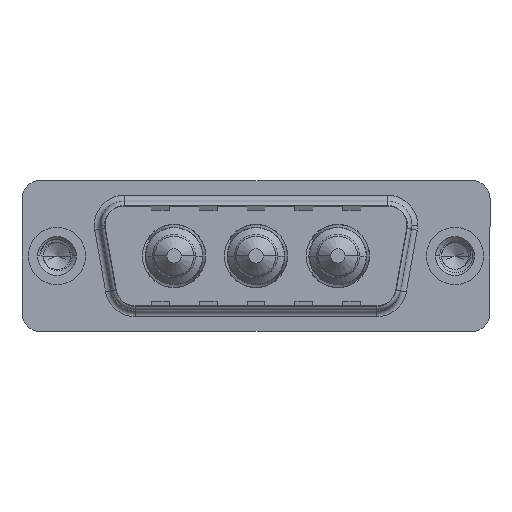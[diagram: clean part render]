
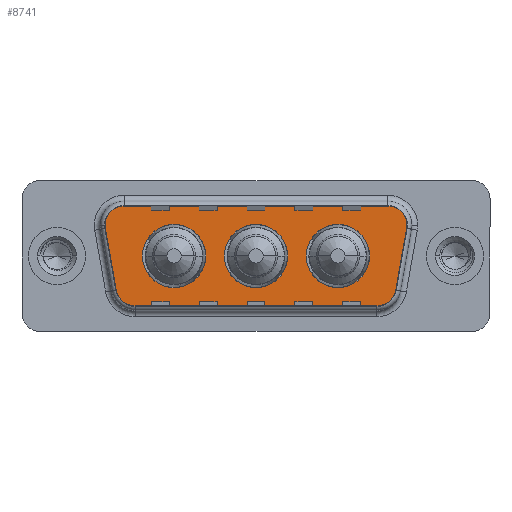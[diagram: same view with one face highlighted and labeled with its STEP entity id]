
A CAD part, top view. The second image highlights one B-rep face of the part: STEP entity #8741.
In plain terms, the highlighted planar face has unit normal (0, 0, 1).
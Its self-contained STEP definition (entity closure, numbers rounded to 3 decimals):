
#190 = CARTESIAN_POINT ( 'NONE',  ( 19.3, 0., 0. ) ) ;
#378 = DIRECTION ( 'NONE',  ( 1., 0., 0. ) ) ;
#458 = ORIENTED_EDGE ( 'NONE', *, *, #9914, .T. ) ;
#621 = VERTEX_POINT ( 'NONE', #1426 ) ;
#658 = LINE ( 'NONE', #4299, #10879 ) ;
#690 = DIRECTION ( 'NONE',  ( 0.174, -0.985, 0. ) ) ;
#710 = CARTESIAN_POINT ( 'NONE',  ( 16.65, 0., 0. ) ) ;
#801 = CARTESIAN_POINT ( 'NONE',  ( 5.411, 2.9, 0. ) ) ;
#1151 = CARTESIAN_POINT ( 'NONE',  ( 26.866, -2.9, 0. ) ) ;
#1298 = AXIS2_PLACEMENT_3D ( 'NONE', #11252, #2921, #12631 ) ;
#1360 = VECTOR ( 'NONE', #6233, 1000. ) ;
#1426 = CARTESIAN_POINT ( 'NONE',  ( 3.441, 2.553, 0. ) ) ;
#1449 = CARTESIAN_POINT ( 'NONE',  ( 27.889, 2.9, 0. ) ) ;
#1453 = VERTEX_POINT ( 'NONE', #14116 ) ;
#1493 = EDGE_CURVE ( 'NONE', #16702, #14204, #7532, .T. ) ;
#1863 = LINE ( 'NONE', #9044, #16305 ) ;
#2009 = CIRCLE ( 'NONE', #5411, 2.65 ) ;
#2084 = CARTESIAN_POINT ( 'NONE',  ( 16.65, 0., 0. ) ) ;
#2113 = ORIENTED_EDGE ( 'NONE', *, *, #17236, .T. ) ;
#2204 = DIRECTION ( 'NONE',  ( 1., 0., 0. ) ) ;
#2831 = DIRECTION ( 'NONE',  ( -1., 0., 0. ) ) ;
#2879 = VERTEX_POINT ( 'NONE', #17013 ) ;
#2913 = AXIS2_PLACEMENT_3D ( 'NONE', #4550, #14225, #5935 ) ;
#2921 = DIRECTION ( 'NONE',  ( 0., 0., 1. ) ) ;
#3236 = CARTESIAN_POINT ( 'NONE',  ( 4.464, -3.247, 0. ) ) ;
#3261 = ORIENTED_EDGE ( 'NONE', *, *, #8033, .T. ) ;
#3480 = AXIS2_PLACEMENT_3D ( 'NONE', #12303, #3997, #13688 ) ;
#3515 = CIRCLE ( 'NONE', #6598, 2. ) ;
#3562 = AXIS2_PLACEMENT_3D ( 'NONE', #13715, #13669, #4082 ) ;
#3754 = ORIENTED_EDGE ( 'NONE', *, *, #13810, .T. ) ;
#3919 = FACE_BOUND ( 'NONE', #4294, .T. ) ;
#3942 = DIRECTION ( 'NONE',  ( 1., 0., 0. ) ) ;
#3997 = DIRECTION ( 'NONE',  ( 0., 0., 1. ) ) ;
#4053 = CIRCLE ( 'NONE', #2913, 2.65 ) ;
#4074 = ORIENTED_EDGE ( 'NONE', *, *, #1493, .F. ) ;
#4082 = DIRECTION ( 'NONE',  ( -1., 0., 0. ) ) ;
#4184 = CARTESIAN_POINT ( 'NONE',  ( 14., 0., 0. ) ) ;
#4294 = EDGE_LOOP ( 'NONE', ( #17870, #17632 ) ) ;
#4298 = AXIS2_PLACEMENT_3D ( 'NONE', #1151, #12256, #3942 ) ;
#4299 = CARTESIAN_POINT ( 'NONE',  ( 5.411, 4.9, 0. ) ) ;
#4375 = VERTEX_POINT ( 'NONE', #16541 ) ;
#4550 = CARTESIAN_POINT ( 'NONE',  ( 23.5, 0., 0. ) ) ;
#4744 = EDGE_CURVE ( 'NONE', #10554, #16624, #2009, .T. ) ;
#4814 = VECTOR ( 'NONE', #14284, 1000. ) ;
#4839 = CARTESIAN_POINT ( 'NONE',  ( 29.889, 2.9, 0. ) ) ;
#5411 = AXIS2_PLACEMENT_3D ( 'NONE', #11672, #6466, #12498 ) ;
#5665 = CIRCLE ( 'NONE', #12994, 2. ) ;
#5678 = DIRECTION ( 'NONE',  ( -1., 0., 0. ) ) ;
#5691 = ORIENTED_EDGE ( 'NONE', *, *, #6945, .F. ) ;
#5935 = DIRECTION ( 'NONE',  ( 1., 0., 0. ) ) ;
#6048 = VERTEX_POINT ( 'NONE', #3236 ) ;
#6144 = CARTESIAN_POINT ( 'NONE',  ( 6.434, -4.9, 0. ) ) ;
#6233 = DIRECTION ( 'NONE',  ( 1., 0., 0. ) ) ;
#6466 = DIRECTION ( 'NONE',  ( 0., 0., 1. ) ) ;
#6551 = CIRCLE ( 'NONE', #9981, 2.65 ) ;
#6598 = AXIS2_PLACEMENT_3D ( 'NONE', #1449, #11163, #2831 ) ;
#6608 = AXIS2_PLACEMENT_3D ( 'NONE', #15687, #7431, #17044 ) ;
#6797 = DIRECTION ( 'NONE',  ( 1., 0., 0. ) ) ;
#6945 = EDGE_CURVE ( 'NONE', #14204, #16702, #16924, .T. ) ;
#6962 = EDGE_CURVE ( 'NONE', #6048, #12454, #16498, .T. ) ;
#7076 = EDGE_CURVE ( 'NONE', #12454, #1453, #12014, .T. ) ;
#7280 = VERTEX_POINT ( 'NONE', #16269 ) ;
#7431 = DIRECTION ( 'NONE',  ( 0., 0., 1. ) ) ;
#7532 = CIRCLE ( 'NONE', #12668, 2.65 ) ;
#7637 = FACE_BOUND ( 'NONE', #17584, .T. ) ;
#7972 = EDGE_CURVE ( 'NONE', #14634, #7280, #6551, .T. ) ;
#8033 = EDGE_CURVE ( 'NONE', #14197, #2879, #12622, .T. ) ;
#8047 = CIRCLE ( 'NONE', #6608, 2. ) ;
#8147 = VERTEX_POINT ( 'NONE', #4839 ) ;
#8609 = EDGE_CURVE ( 'NONE', #4375, #621, #5665, .T. ) ;
#8741 = ADVANCED_FACE ( 'NONE', ( #7637, #11755, #3919, #14968 ), #10873, .T. ) ;
#8758 = DIRECTION ( 'NONE',  ( 0., 0., 1. ) ) ;
#9044 = CARTESIAN_POINT ( 'NONE',  ( 3.441, 2.553, 0. ) ) ;
#9218 = EDGE_LOOP ( 'NONE', ( #458, #3261, #12146, #12480, #2113, #16276, #3754, #17458, #13937 ) ) ;
#9914 = EDGE_CURVE ( 'NONE', #1453, #14197, #8047, .T. ) ;
#9981 = AXIS2_PLACEMENT_3D ( 'NONE', #16967, #8758, #378 ) ;
#10226 = EDGE_CURVE ( 'NONE', #16624, #10554, #11932, .T. ) ;
#10470 = EDGE_LOOP ( 'NONE', ( #15898, #15599 ) ) ;
#10525 = DIRECTION ( 'NONE',  ( 0., 0., 1. ) ) ;
#10554 = VERTEX_POINT ( 'NONE', #11631 ) ;
#10873 = PLANE ( 'NONE',  #4298 ) ;
#10879 = VECTOR ( 'NONE', #5678, 1000. ) ;
#11163 = DIRECTION ( 'NONE',  ( 0., 0., 1. ) ) ;
#11252 = CARTESIAN_POINT ( 'NONE',  ( 27.889, 2.9, 0. ) ) ;
#11590 = CARTESIAN_POINT ( 'NONE',  ( 29.859, 2.553, 0. ) ) ;
#11631 = CARTESIAN_POINT ( 'NONE',  ( 7.15, 0., 0. ) ) ;
#11672 = CARTESIAN_POINT ( 'NONE',  ( 9.8, 0., 0. ) ) ;
#11755 = FACE_BOUND ( 'NONE', #10470, .T. ) ;
#11932 = CIRCLE ( 'NONE', #3480, 2.65 ) ;
#12014 = LINE ( 'NONE', #6144, #1360 ) ;
#12075 = EDGE_CURVE ( 'NONE', #7280, #14634, #4053, .T. ) ;
#12146 = ORIENTED_EDGE ( 'NONE', *, *, #15267, .T. ) ;
#12226 = CARTESIAN_POINT ( 'NONE',  ( 20.85, 0., 0. ) ) ;
#12256 = DIRECTION ( 'NONE',  ( 0., 0., 1. ) ) ;
#12281 = CIRCLE ( 'NONE', #1298, 2. ) ;
#12303 = CARTESIAN_POINT ( 'NONE',  ( 9.8, 0., 0. ) ) ;
#12454 = VERTEX_POINT ( 'NONE', #13655 ) ;
#12480 = ORIENTED_EDGE ( 'NONE', *, *, #12642, .T. ) ;
#12498 = DIRECTION ( 'NONE',  ( 1., 0., 0. ) ) ;
#12622 = LINE ( 'NONE', #11590, #4814 ) ;
#12631 = DIRECTION ( 'NONE',  ( -1., 0., 0. ) ) ;
#12642 = EDGE_CURVE ( 'NONE', #8147, #12751, #12281, .T. ) ;
#12668 = AXIS2_PLACEMENT_3D ( 'NONE', #710, #15095, #6797 ) ;
#12751 = VERTEX_POINT ( 'NONE', #14196 ) ;
#12994 = AXIS2_PLACEMENT_3D ( 'NONE', #801, #10525, #2204 ) ;
#13655 = CARTESIAN_POINT ( 'NONE',  ( 6.434, -4.9, 0. ) ) ;
#13669 = DIRECTION ( 'NONE',  ( 0., 0., 1. ) ) ;
#13688 = DIRECTION ( 'NONE',  ( 1., 0., 0. ) ) ;
#13715 = CARTESIAN_POINT ( 'NONE',  ( 6.434, -2.9, 0. ) ) ;
#13810 = EDGE_CURVE ( 'NONE', #621, #6048, #1863, .T. ) ;
#13867 = CARTESIAN_POINT ( 'NONE',  ( 28.836, -3.247, 0. ) ) ;
#13937 = ORIENTED_EDGE ( 'NONE', *, *, #7076, .T. ) ;
#14116 = CARTESIAN_POINT ( 'NONE',  ( 26.866, -4.9, 0. ) ) ;
#14196 = CARTESIAN_POINT ( 'NONE',  ( 27.889, 4.9, 0. ) ) ;
#14197 = VERTEX_POINT ( 'NONE', #13867 ) ;
#14204 = VERTEX_POINT ( 'NONE', #4184 ) ;
#14225 = DIRECTION ( 'NONE',  ( 0., 0., 1. ) ) ;
#14284 = DIRECTION ( 'NONE',  ( 0.174, 0.985, 0. ) ) ;
#14490 = DIRECTION ( 'NONE',  ( 1., 0., 0. ) ) ;
#14610 = DIRECTION ( 'NONE',  ( 0., 0., 1. ) ) ;
#14634 = VERTEX_POINT ( 'NONE', #12226 ) ;
#14968 = FACE_OUTER_BOUND ( 'NONE', #9218, .T. ) ;
#15095 = DIRECTION ( 'NONE',  ( 0., 0., 1. ) ) ;
#15267 = EDGE_CURVE ( 'NONE', #2879, #8147, #3515, .T. ) ;
#15599 = ORIENTED_EDGE ( 'NONE', *, *, #7972, .F. ) ;
#15687 = CARTESIAN_POINT ( 'NONE',  ( 26.866, -2.9, 0. ) ) ;
#15898 = ORIENTED_EDGE ( 'NONE', *, *, #12075, .F. ) ;
#16269 = CARTESIAN_POINT ( 'NONE',  ( 26.15, 0., 0. ) ) ;
#16276 = ORIENTED_EDGE ( 'NONE', *, *, #8609, .T. ) ;
#16305 = VECTOR ( 'NONE', #690, 1000. ) ;
#16498 = CIRCLE ( 'NONE', #3562, 2. ) ;
#16541 = CARTESIAN_POINT ( 'NONE',  ( 5.411, 4.9, 0. ) ) ;
#16624 = VERTEX_POINT ( 'NONE', #16672 ) ;
#16672 = CARTESIAN_POINT ( 'NONE',  ( 12.45, 0., 0. ) ) ;
#16702 = VERTEX_POINT ( 'NONE', #190 ) ;
#16851 = AXIS2_PLACEMENT_3D ( 'NONE', #2084, #14610, #14490 ) ;
#16924 = CIRCLE ( 'NONE', #16851, 2.65 ) ;
#16967 = CARTESIAN_POINT ( 'NONE',  ( 23.5, 0., 0. ) ) ;
#17013 = CARTESIAN_POINT ( 'NONE',  ( 29.859, 2.553, 0. ) ) ;
#17044 = DIRECTION ( 'NONE',  ( 1., 0., 0. ) ) ;
#17236 = EDGE_CURVE ( 'NONE', #12751, #4375, #658, .T. ) ;
#17458 = ORIENTED_EDGE ( 'NONE', *, *, #6962, .T. ) ;
#17584 = EDGE_LOOP ( 'NONE', ( #4074, #5691 ) ) ;
#17632 = ORIENTED_EDGE ( 'NONE', *, *, #4744, .F. ) ;
#17870 = ORIENTED_EDGE ( 'NONE', *, *, #10226, .F. ) ;
